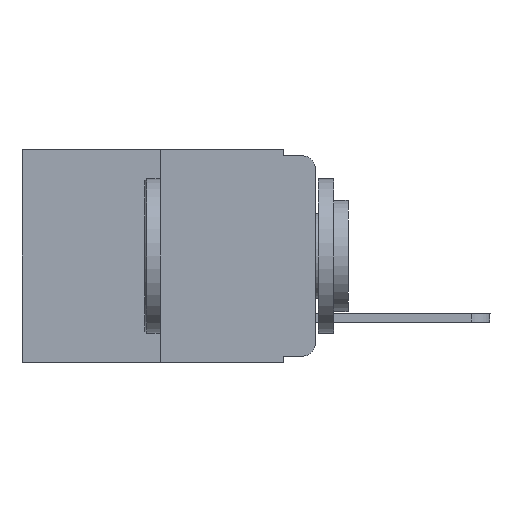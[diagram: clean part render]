
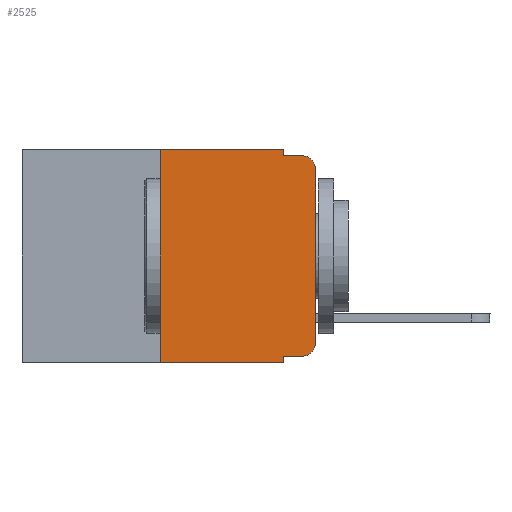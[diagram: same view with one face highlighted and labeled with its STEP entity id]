
A CAD part, left-side view. The second image highlights one B-rep face of the part: STEP entity #2525.
In plain terms, the highlighted planar face has unit normal (-1, 0, 0).
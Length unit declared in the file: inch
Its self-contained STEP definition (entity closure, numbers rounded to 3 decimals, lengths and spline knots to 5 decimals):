
#135 = EDGE_CURVE ( 'NONE', #12821, #166, #10949, .T. ) ;
#166 = VERTEX_POINT ( 'NONE', #2594 ) ;
#782 = DIRECTION ( 'NONE',  ( 0., -1., 0. ) ) ;
#876 = DIRECTION ( 'NONE',  ( 1., 0., 0. ) ) ;
#878 = CARTESIAN_POINT ( 'NONE',  ( 0., 0.051, -0.333 ) ) ;
#911 = EDGE_CURVE ( 'NONE', #10186, #4050, #6012, .T. ) ;
#1056 = LINE ( 'NONE', #8184, #11137 ) ;
#1162 = DIRECTION ( 'NONE',  ( 0., 0., -1. ) ) ;
#1246 = DIRECTION ( 'NONE',  ( 0., 0., 1. ) ) ;
#1358 = CARTESIAN_POINT ( 'NONE',  ( 0., 0.051, -0.333 ) ) ;
#1379 = ORIENTED_EDGE ( 'NONE', *, *, #11059, .F. ) ;
#1386 = EDGE_CURVE ( 'NONE', #4050, #9678, #2754, .T. ) ;
#1760 = CARTESIAN_POINT ( 'NONE',  ( 0., 0.051, -0.343 ) ) ;
#1777 = VERTEX_POINT ( 'NONE', #2694 ) ;
#2244 = DIRECTION ( 'NONE',  ( 0., 0., -1. ) ) ;
#2370 = DIRECTION ( 'NONE',  ( 0., 0., 1. ) ) ;
#2451 = CARTESIAN_POINT ( 'NONE',  ( 0., 0.051, 0. ) ) ;
#2525 = ADVANCED_FACE ( 'NONE', ( #12603 ), #6893, .F. ) ;
#2594 = CARTESIAN_POINT ( 'NONE',  ( 0., 0.051, 0. ) ) ;
#2609 = ORIENTED_EDGE ( 'NONE', *, *, #135, .F. ) ;
#2694 = CARTESIAN_POINT ( 'NONE',  ( 0., 0.02, -0.01 ) ) ;
#2754 = LINE ( 'NONE', #2892, #3385 ) ;
#2865 = CARTESIAN_POINT ( 'NONE',  ( 0., 0., -0.313 ) ) ;
#2892 = CARTESIAN_POINT ( 'NONE',  ( 0., 0., 0. ) ) ;
#3095 = DIRECTION ( 'NONE',  ( -1., 0., 0. ) ) ;
#3182 = ORIENTED_EDGE ( 'NONE', *, *, #10423, .T. ) ;
#3385 = VECTOR ( 'NONE', #1246, 39.37008 ) ;
#3769 = LINE ( 'NONE', #2451, #8684 ) ;
#4038 = CARTESIAN_POINT ( 'NONE',  ( 0., 0.051, -0.01 ) ) ;
#4050 = VERTEX_POINT ( 'NONE', #2865 ) ;
#4136 = ORIENTED_EDGE ( 'NONE', *, *, #4665, .F. ) ;
#4665 = EDGE_CURVE ( 'NONE', #12102, #1777, #8378, .T. ) ;
#4671 = DIRECTION ( 'NONE',  ( 0., -1., 0. ) ) ;
#4865 = ORIENTED_EDGE ( 'NONE', *, *, #11348, .T. ) ;
#5103 = ORIENTED_EDGE ( 'NONE', *, *, #7870, .T. ) ;
#5166 = EDGE_CURVE ( 'NONE', #166, #12102, #7442, .T. ) ;
#5630 = LINE ( 'NONE', #1358, #6534 ) ;
#5685 = VECTOR ( 'NONE', #4671, 39.37008 ) ;
#5881 = EDGE_LOOP ( 'NONE', ( #6549, #4865, #4136, #10192, #2609, #12234, #5103, #1379, #3182, #6929 ) ) ;
#6012 = CIRCLE ( 'NONE', #9702, 0.02 ) ;
#6130 = CARTESIAN_POINT ( 'NONE',  ( 0., 0.051, -0.01 ) ) ;
#6163 = CARTESIAN_POINT ( 'NONE',  ( 0., 0.051, 0. ) ) ;
#6224 = DIRECTION ( 'NONE',  ( -1., 0., 0. ) ) ;
#6358 = CIRCLE ( 'NONE', #7876, 0.02 ) ;
#6534 = VECTOR ( 'NONE', #7344, 39.37008 ) ;
#6549 = ORIENTED_EDGE ( 'NONE', *, *, #1386, .T. ) ;
#6883 = DIRECTION ( 'NONE',  ( 0., 0., -1. ) ) ;
#6888 = VERTEX_POINT ( 'NONE', #12095 ) ;
#6893 = PLANE ( 'NONE',  #11528 ) ;
#6929 = ORIENTED_EDGE ( 'NONE', *, *, #911, .T. ) ;
#7094 = CARTESIAN_POINT ( 'NONE',  ( 0., 0., -0.03 ) ) ;
#7183 = CARTESIAN_POINT ( 'NONE',  ( 0., 0.02, -0.313 ) ) ;
#7344 = DIRECTION ( 'NONE',  ( 0., -1., 0. ) ) ;
#7442 = LINE ( 'NONE', #6163, #8981 ) ;
#7673 = LINE ( 'NONE', #12580, #11845 ) ;
#7870 = EDGE_CURVE ( 'NONE', #6888, #10742, #7673, .T. ) ;
#7876 = AXIS2_PLACEMENT_3D ( 'NONE', #11816, #3095, #6883 ) ;
#7916 = CARTESIAN_POINT ( 'NONE',  ( 0., 0.02, -0.333 ) ) ;
#7917 = DIRECTION ( 'NONE',  ( 0., -1., 0. ) ) ;
#8184 = CARTESIAN_POINT ( 'NONE',  ( 0., 0.25, 0. ) ) ;
#8378 = LINE ( 'NONE', #4038, #11175 ) ;
#8684 = VECTOR ( 'NONE', #9356, 39.37008 ) ;
#8811 = VERTEX_POINT ( 'NONE', #878 ) ;
#8981 = VECTOR ( 'NONE', #2244, 39.37008 ) ;
#9356 = DIRECTION ( 'NONE',  ( 0., 0., -1. ) ) ;
#9678 = VERTEX_POINT ( 'NONE', #7094 ) ;
#9702 = AXIS2_PLACEMENT_3D ( 'NONE', #7183, #6224, #1162 ) ;
#9848 = DIRECTION ( 'NONE',  ( 0., 0., -1. ) ) ;
#10186 = VERTEX_POINT ( 'NONE', #7916 ) ;
#10192 = ORIENTED_EDGE ( 'NONE', *, *, #5166, .F. ) ;
#10376 = CARTESIAN_POINT ( 'NONE',  ( 0., 0.473, 0. ) ) ;
#10423 = EDGE_CURVE ( 'NONE', #8811, #10186, #5630, .T. ) ;
#10742 = VERTEX_POINT ( 'NONE', #1760 ) ;
#10949 = LINE ( 'NONE', #10376, #5685 ) ;
#11059 = EDGE_CURVE ( 'NONE', #8811, #10742, #3769, .T. ) ;
#11137 = VECTOR ( 'NONE', #2370, 39.37008 ) ;
#11175 = VECTOR ( 'NONE', #7917, 39.37008 ) ;
#11348 = EDGE_CURVE ( 'NONE', #9678, #1777, #6358, .T. ) ;
#11360 = CARTESIAN_POINT ( 'NONE',  ( 0., 0.25, 0. ) ) ;
#11528 = AXIS2_PLACEMENT_3D ( 'NONE', #11741, #876, #9848 ) ;
#11741 = CARTESIAN_POINT ( 'NONE',  ( 0., 0.473, 0. ) ) ;
#11816 = CARTESIAN_POINT ( 'NONE',  ( 0., 0.02, -0.03 ) ) ;
#11845 = VECTOR ( 'NONE', #782, 39.37008 ) ;
#12095 = CARTESIAN_POINT ( 'NONE',  ( 0., 0.25, -0.343 ) ) ;
#12102 = VERTEX_POINT ( 'NONE', #6130 ) ;
#12234 = ORIENTED_EDGE ( 'NONE', *, *, #12707, .F. ) ;
#12580 = CARTESIAN_POINT ( 'NONE',  ( 0., 0.473, -0.343 ) ) ;
#12603 = FACE_OUTER_BOUND ( 'NONE', #5881, .T. ) ;
#12707 = EDGE_CURVE ( 'NONE', #6888, #12821, #1056, .T. ) ;
#12821 = VERTEX_POINT ( 'NONE', #11360 ) ;
